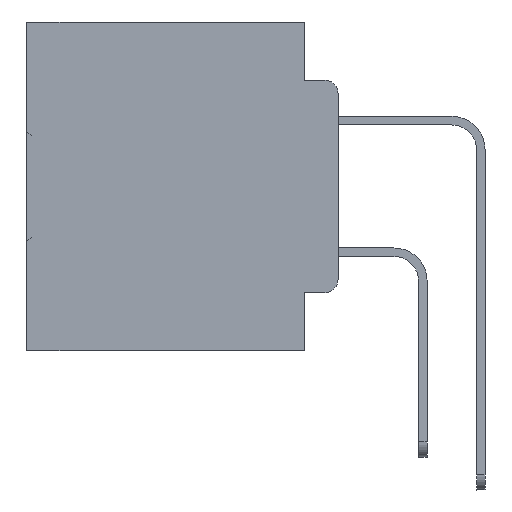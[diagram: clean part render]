
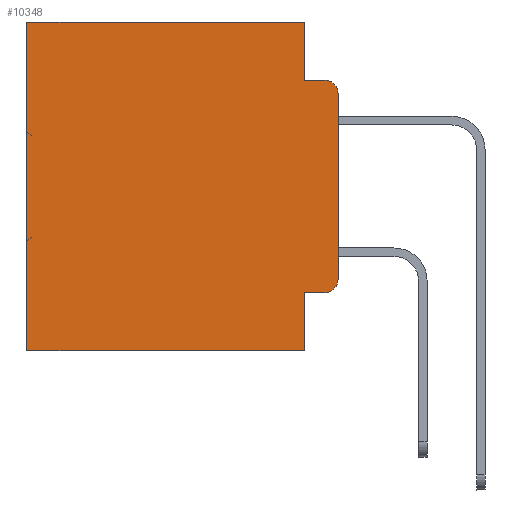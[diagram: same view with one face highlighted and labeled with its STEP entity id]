
A CAD part, left-side view. The second image highlights one B-rep face of the part: STEP entity #10348.
In plain terms, the highlighted planar face has unit normal (-1, 0, 0).
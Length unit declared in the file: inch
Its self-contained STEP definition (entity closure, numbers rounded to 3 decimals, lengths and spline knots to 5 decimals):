
#580 = CARTESIAN_POINT ( 'NONE',  ( 0.298, 0., -0.3915 ) ) ;
#593 = DIRECTION ( 'NONE',  ( 0., 0., -1. ) ) ;
#891 = CARTESIAN_POINT ( 'NONE',  ( 0.298, 0., 0. ) ) ;
#939 = ORIENTED_EDGE ( 'NONE', *, *, #28765, .F. ) ;
#1815 = EDGE_CURVE ( 'NONE', #32878, #25213, #3437, .T. ) ;
#2173 = VERTEX_POINT ( 'NONE', #19059 ) ;
#2469 = DIRECTION ( 'NONE',  ( 0., 1., 0. ) ) ;
#3239 = VECTOR ( 'NONE', #13072, 39.37008 ) ;
#3335 = EDGE_CURVE ( 'NONE', #16786, #25213, #11481, .T. ) ;
#3437 = CIRCLE ( 'NONE', #32089, 0.02 ) ;
#3479 = EDGE_CURVE ( 'NONE', #2173, #19615, #9144, .T. ) ;
#3646 = DIRECTION ( 'NONE',  ( 0., 1., 0. ) ) ;
#4271 = CARTESIAN_POINT ( 'NONE',  ( 0.298, 0.02, -0.1085 ) ) ;
#4817 = CARTESIAN_POINT ( 'NONE',  ( 0.298, 0.051, 0. ) ) ;
#5374 = CARTESIAN_POINT ( 'NONE',  ( 0.298, 0.051, -0.0885 ) ) ;
#6352 = DIRECTION ( 'NONE',  ( 0., 0., -1. ) ) ;
#8840 = CARTESIAN_POINT ( 'NONE',  ( 0.298, 0., -0.1085 ) ) ;
#8906 = CARTESIAN_POINT ( 'NONE',  ( 0.298, 0., 0. ) ) ;
#9144 = LINE ( 'NONE', #36036, #21897 ) ;
#10348 = ADVANCED_FACE ( 'NONE', ( #14974 ), #26843, .F. ) ;
#10797 = VECTOR ( 'NONE', #18247, 39.37008 ) ;
#11481 = LINE ( 'NONE', #29241, #35562 ) ;
#12016 = ORIENTED_EDGE ( 'NONE', *, *, #38196, .T. ) ;
#12586 = ORIENTED_EDGE ( 'NONE', *, *, #30690, .F. ) ;
#12945 = CARTESIAN_POINT ( 'NONE',  ( 0.298, 0.02, -0.4115 ) ) ;
#13072 = DIRECTION ( 'NONE',  ( 0., 0., -1. ) ) ;
#13875 = CARTESIAN_POINT ( 'NONE',  ( 0.298, 0.051, 0. ) ) ;
#14086 = VECTOR ( 'NONE', #16934, 39.37008 ) ;
#14207 = LINE ( 'NONE', #4817, #10797 ) ;
#14974 = FACE_OUTER_BOUND ( 'NONE', #27522, .T. ) ;
#16163 = VERTEX_POINT ( 'NONE', #580 ) ;
#16637 = CARTESIAN_POINT ( 'NONE',  ( 0.298, 0.02, -0.0885 ) ) ;
#16718 = ORIENTED_EDGE ( 'NONE', *, *, #29484, .F. ) ;
#16786 = VERTEX_POINT ( 'NONE', #5374 ) ;
#16934 = DIRECTION ( 'NONE',  ( 0., 0., -1. ) ) ;
#18247 = DIRECTION ( 'NONE',  ( 0., 0., -1. ) ) ;
#19059 = CARTESIAN_POINT ( 'NONE',  ( 0.298, 0.051, -0.4115 ) ) ;
#19565 = DIRECTION ( 'NONE',  ( 0., 0., -1. ) ) ;
#19615 = VERTEX_POINT ( 'NONE', #12945 ) ;
#19708 = CARTESIAN_POINT ( 'NONE',  ( 0.298, 0.051, 0. ) ) ;
#20224 = LINE ( 'NONE', #37237, #24535 ) ;
#21606 = ORIENTED_EDGE ( 'NONE', *, *, #34491, .T. ) ;
#21897 = VECTOR ( 'NONE', #23760, 39.37008 ) ;
#22638 = VECTOR ( 'NONE', #593, 39.37008 ) ;
#22774 = LINE ( 'NONE', #31742, #14086 ) ;
#22823 = CIRCLE ( 'NONE', #34019, 0.02 ) ;
#23283 = ORIENTED_EDGE ( 'NONE', *, *, #34102, .F. ) ;
#23760 = DIRECTION ( 'NONE',  ( 0., -1., 0. ) ) ;
#24407 = LINE ( 'NONE', #24793, #22638 ) ;
#24535 = VECTOR ( 'NONE', #2469, 39.37008 ) ;
#24548 = DIRECTION ( 'NONE',  ( -1., 0., 0. ) ) ;
#24705 = LINE ( 'NONE', #891, #35555 ) ;
#24742 = DIRECTION ( 'NONE',  ( 0., 0., -1. ) ) ;
#24757 = LINE ( 'NONE', #19708, #3239 ) ;
#24793 = CARTESIAN_POINT ( 'NONE',  ( 0.298, 0.473, 0. ) ) ;
#25213 = VERTEX_POINT ( 'NONE', #16637 ) ;
#25252 = CARTESIAN_POINT ( 'NONE',  ( 0.298, 0.051, -0.5 ) ) ;
#26170 = DIRECTION ( 'NONE',  ( -1., 0., 0. ) ) ;
#26843 = PLANE ( 'NONE',  #28353 ) ;
#27038 = DIRECTION ( 'NONE',  ( 1., 0., 0. ) ) ;
#27522 = EDGE_LOOP ( 'NONE', ( #23283, #35431, #36184, #16718, #33098, #12016, #12586, #939, #29644, #21606 ) ) ;
#27832 = EDGE_CURVE ( 'NONE', #35047, #31180, #24705, .T. ) ;
#28353 = AXIS2_PLACEMENT_3D ( 'NONE', #8906, #27038, #6352 ) ;
#28765 = EDGE_CURVE ( 'NONE', #2173, #32609, #24757, .T. ) ;
#28820 = VERTEX_POINT ( 'NONE', #33923 ) ;
#29241 = CARTESIAN_POINT ( 'NONE',  ( 0.298, 0.051, -0.0885 ) ) ;
#29484 = EDGE_CURVE ( 'NONE', #35047, #16786, #14207, .T. ) ;
#29644 = ORIENTED_EDGE ( 'NONE', *, *, #3479, .T. ) ;
#30690 = EDGE_CURVE ( 'NONE', #32609, #28820, #20224, .T. ) ;
#31180 = VERTEX_POINT ( 'NONE', #34424 ) ;
#31742 = CARTESIAN_POINT ( 'NONE',  ( 0.298, 0., 0. ) ) ;
#32089 = AXIS2_PLACEMENT_3D ( 'NONE', #4271, #24548, #24742 ) ;
#32609 = VERTEX_POINT ( 'NONE', #25252 ) ;
#32878 = VERTEX_POINT ( 'NONE', #8840 ) ;
#33098 = ORIENTED_EDGE ( 'NONE', *, *, #27832, .T. ) ;
#33923 = CARTESIAN_POINT ( 'NONE',  ( 0.298, 0.473, -0.5 ) ) ;
#34019 = AXIS2_PLACEMENT_3D ( 'NONE', #37881, #26170, #19565 ) ;
#34102 = EDGE_CURVE ( 'NONE', #32878, #16163, #22774, .T. ) ;
#34424 = CARTESIAN_POINT ( 'NONE',  ( 0.298, 0.473, 0. ) ) ;
#34491 = EDGE_CURVE ( 'NONE', #19615, #16163, #22823, .T. ) ;
#35047 = VERTEX_POINT ( 'NONE', #13875 ) ;
#35431 = ORIENTED_EDGE ( 'NONE', *, *, #1815, .T. ) ;
#35555 = VECTOR ( 'NONE', #3646, 39.37008 ) ;
#35562 = VECTOR ( 'NONE', #38016, 39.37008 ) ;
#36036 = CARTESIAN_POINT ( 'NONE',  ( 0.298, 0.051, -0.4115 ) ) ;
#36184 = ORIENTED_EDGE ( 'NONE', *, *, #3335, .F. ) ;
#37237 = CARTESIAN_POINT ( 'NONE',  ( 0.298, 0., -0.5 ) ) ;
#37881 = CARTESIAN_POINT ( 'NONE',  ( 0.298, 0.02, -0.3915 ) ) ;
#38016 = DIRECTION ( 'NONE',  ( 0., -1., 0. ) ) ;
#38196 = EDGE_CURVE ( 'NONE', #31180, #28820, #24407, .T. ) ;
